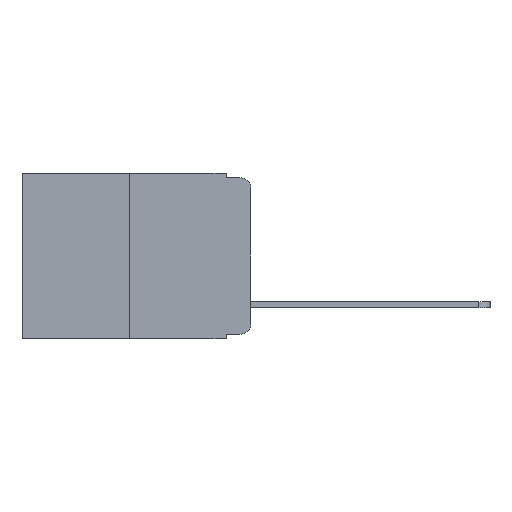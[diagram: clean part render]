
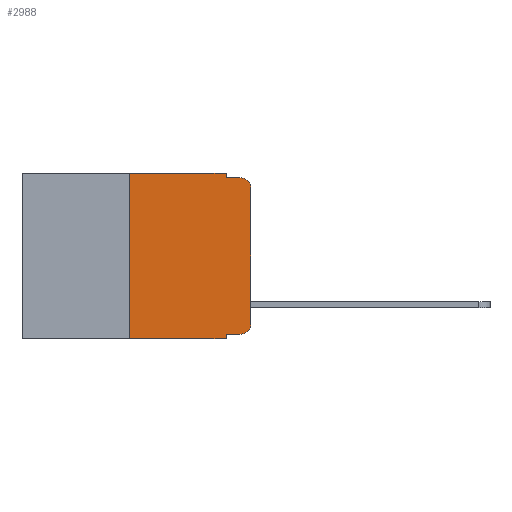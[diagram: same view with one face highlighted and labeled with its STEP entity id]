
A CAD part, left-side view. The second image highlights one B-rep face of the part: STEP entity #2988.
In plain terms, the highlighted planar face has unit normal (-1, 0, 0).
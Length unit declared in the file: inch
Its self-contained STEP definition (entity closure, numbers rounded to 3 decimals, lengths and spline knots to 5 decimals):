
#129 = EDGE_CURVE ( 'NONE', #1560, #3087, #1881, .T. ) ;
#239 = CARTESIAN_POINT ( 'NONE',  ( 0., 0.473, 0. ) ) ;
#251 = DIRECTION ( 'NONE',  ( 1., 0., 0. ) ) ;
#353 = DIRECTION ( 'NONE',  ( 0., 0., 1. ) ) ;
#463 = PLANE ( 'NONE',  #4961 ) ;
#710 = ORIENTED_EDGE ( 'NONE', *, *, #7308, .T. ) ;
#773 = EDGE_CURVE ( 'NONE', #10764, #3087, #9867, .T. ) ;
#848 = FACE_OUTER_BOUND ( 'NONE', #4010, .T. ) ;
#883 = ORIENTED_EDGE ( 'NONE', *, *, #4816, .F. ) ;
#957 = LINE ( 'NONE', #9088, #6175 ) ;
#1235 = ORIENTED_EDGE ( 'NONE', *, *, #6123, .F. ) ;
#1245 = VECTOR ( 'NONE', #8163, 39.37008 ) ;
#1420 = DIRECTION ( 'NONE',  ( 0., -1., 0. ) ) ;
#1467 = VERTEX_POINT ( 'NONE', #6834 ) ;
#1560 = VERTEX_POINT ( 'NONE', #11108 ) ;
#1881 = CIRCLE ( 'NONE', #3281, 0.02 ) ;
#1950 = DIRECTION ( 'NONE',  ( 0., -1., 0. ) ) ;
#2006 = CARTESIAN_POINT ( 'NONE',  ( 0., 0.25, -0.343 ) ) ;
#2067 = DIRECTION ( 'NONE',  ( -1., 0., 0. ) ) ;
#2250 = VERTEX_POINT ( 'NONE', #10612 ) ;
#2264 = VERTEX_POINT ( 'NONE', #6570 ) ;
#2329 = ORIENTED_EDGE ( 'NONE', *, *, #3898, .T. ) ;
#2560 = ORIENTED_EDGE ( 'NONE', *, *, #2786, .F. ) ;
#2631 = VECTOR ( 'NONE', #1950, 39.37008 ) ;
#2721 = CARTESIAN_POINT ( 'NONE',  ( 0., 0.473, -0.343 ) ) ;
#2786 = EDGE_CURVE ( 'NONE', #9687, #10764, #11084, .T. ) ;
#2926 = CARTESIAN_POINT ( 'NONE',  ( 0., 0.051, 0. ) ) ;
#2988 = ADVANCED_FACE ( 'NONE', ( #848 ), #463, .F. ) ;
#3087 = VERTEX_POINT ( 'NONE', #9955 ) ;
#3179 = VERTEX_POINT ( 'NONE', #9472 ) ;
#3281 = AXIS2_PLACEMENT_3D ( 'NONE', #11437, #11473, #10916 ) ;
#3312 = CARTESIAN_POINT ( 'NONE',  ( 0., 0.02, -0.333 ) ) ;
#3415 = ORIENTED_EDGE ( 'NONE', *, *, #6664, .T. ) ;
#3491 = EDGE_CURVE ( 'NONE', #10336, #1467, #4920, .T. ) ;
#3562 = ORIENTED_EDGE ( 'NONE', *, *, #10565, .T. ) ;
#3898 = EDGE_CURVE ( 'NONE', #10336, #2250, #9500, .T. ) ;
#3945 = LINE ( 'NONE', #11533, #1245 ) ;
#4010 = EDGE_LOOP ( 'NONE', ( #3562, #9532, #10124, #2560, #1235, #11106, #2329, #883, #3415, #710 ) ) ;
#4477 = DIRECTION ( 'NONE',  ( 0., 0., -1. ) ) ;
#4816 = EDGE_CURVE ( 'NONE', #2264, #2250, #957, .T. ) ;
#4910 = VECTOR ( 'NONE', #1420, 39.37008 ) ;
#4920 = LINE ( 'NONE', #6661, #7093 ) ;
#4961 = AXIS2_PLACEMENT_3D ( 'NONE', #239, #251, #7019 ) ;
#5106 = CIRCLE ( 'NONE', #9200, 0.02 ) ;
#5285 = CARTESIAN_POINT ( 'NONE',  ( 0., 0., 0. ) ) ;
#5844 = CARTESIAN_POINT ( 'NONE',  ( 0., 0.051, -0.333 ) ) ;
#6027 = CARTESIAN_POINT ( 'NONE',  ( 0., 0.051, 0. ) ) ;
#6086 = CARTESIAN_POINT ( 'NONE',  ( 0., 0.051, -0.01 ) ) ;
#6123 = EDGE_CURVE ( 'NONE', #1467, #9687, #3945, .T. ) ;
#6146 = DIRECTION ( 'NONE',  ( 0., -1., 0. ) ) ;
#6175 = VECTOR ( 'NONE', #4477, 39.37008 ) ;
#6570 = CARTESIAN_POINT ( 'NONE',  ( 0., 0.051, -0.333 ) ) ;
#6661 = CARTESIAN_POINT ( 'NONE',  ( 0., 0.25, 0. ) ) ;
#6664 = EDGE_CURVE ( 'NONE', #2264, #11892, #7999, .T. ) ;
#6834 = CARTESIAN_POINT ( 'NONE',  ( 0., 0.25, 0. ) ) ;
#7019 = DIRECTION ( 'NONE',  ( 0., 0., -1. ) ) ;
#7075 = VECTOR ( 'NONE', #353, 39.37008 ) ;
#7093 = VECTOR ( 'NONE', #11970, 39.37008 ) ;
#7308 = EDGE_CURVE ( 'NONE', #11892, #3179, #5106, .T. ) ;
#7786 = CARTESIAN_POINT ( 'NONE',  ( 0., 0.02, -0.313 ) ) ;
#7999 = LINE ( 'NONE', #5844, #2631 ) ;
#8163 = DIRECTION ( 'NONE',  ( 0., -1., 0. ) ) ;
#8722 = DIRECTION ( 'NONE',  ( 0., 0., -1. ) ) ;
#8968 = VECTOR ( 'NONE', #11376, 39.37008 ) ;
#9088 = CARTESIAN_POINT ( 'NONE',  ( 0., 0.051, 0. ) ) ;
#9200 = AXIS2_PLACEMENT_3D ( 'NONE', #7786, #2067, #8722 ) ;
#9472 = CARTESIAN_POINT ( 'NONE',  ( 0., 0., -0.313 ) ) ;
#9500 = LINE ( 'NONE', #2721, #4910 ) ;
#9532 = ORIENTED_EDGE ( 'NONE', *, *, #129, .T. ) ;
#9578 = VECTOR ( 'NONE', #6146, 39.37008 ) ;
#9687 = VERTEX_POINT ( 'NONE', #6027 ) ;
#9867 = LINE ( 'NONE', #6086, #9578 ) ;
#9955 = CARTESIAN_POINT ( 'NONE',  ( 0., 0.02, -0.01 ) ) ;
#10124 = ORIENTED_EDGE ( 'NONE', *, *, #773, .F. ) ;
#10336 = VERTEX_POINT ( 'NONE', #2006 ) ;
#10565 = EDGE_CURVE ( 'NONE', #3179, #1560, #11879, .T. ) ;
#10612 = CARTESIAN_POINT ( 'NONE',  ( 0., 0.051, -0.343 ) ) ;
#10764 = VERTEX_POINT ( 'NONE', #11038 ) ;
#10916 = DIRECTION ( 'NONE',  ( 0., 0., -1. ) ) ;
#11038 = CARTESIAN_POINT ( 'NONE',  ( 0., 0.051, -0.01 ) ) ;
#11084 = LINE ( 'NONE', #2926, #8968 ) ;
#11106 = ORIENTED_EDGE ( 'NONE', *, *, #3491, .F. ) ;
#11108 = CARTESIAN_POINT ( 'NONE',  ( 0., 0., -0.03 ) ) ;
#11376 = DIRECTION ( 'NONE',  ( 0., 0., -1. ) ) ;
#11437 = CARTESIAN_POINT ( 'NONE',  ( 0., 0.02, -0.03 ) ) ;
#11473 = DIRECTION ( 'NONE',  ( -1., 0., 0. ) ) ;
#11533 = CARTESIAN_POINT ( 'NONE',  ( 0., 0.473, 0. ) ) ;
#11879 = LINE ( 'NONE', #5285, #7075 ) ;
#11892 = VERTEX_POINT ( 'NONE', #3312 ) ;
#11970 = DIRECTION ( 'NONE',  ( 0., 0., 1. ) ) ;
